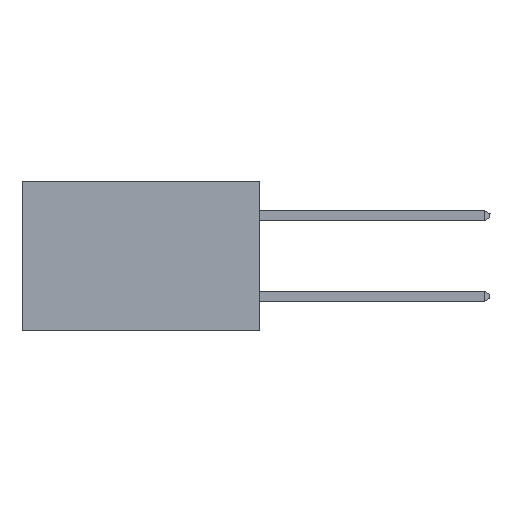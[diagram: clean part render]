
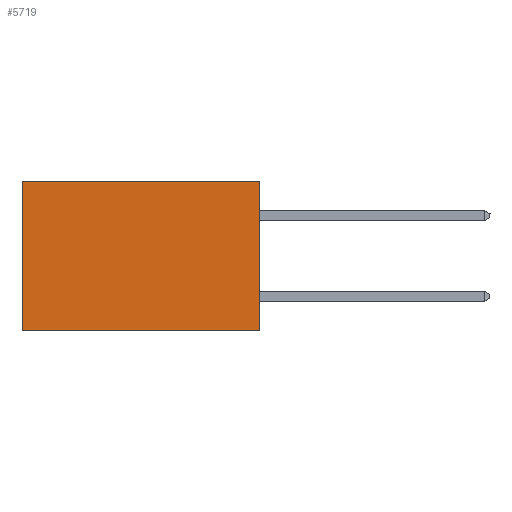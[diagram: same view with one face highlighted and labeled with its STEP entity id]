
A CAD part, left-side view. The second image highlights one B-rep face of the part: STEP entity #5719.
In plain terms, the highlighted planar face has unit normal (-1, 0, 0).
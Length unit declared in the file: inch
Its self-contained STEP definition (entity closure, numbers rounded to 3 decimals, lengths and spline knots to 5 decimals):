
#597 = CARTESIAN_POINT ( 'NONE',  ( 0.277, 0., -0.37 ) ) ;
#754 = LINE ( 'NONE', #7205, #15923 ) ;
#850 = CARTESIAN_POINT ( 'NONE',  ( 0.277, 0., -0.37 ) ) ;
#2019 = DIRECTION ( 'NONE',  ( 0., 1., 0. ) ) ;
#2414 = CARTESIAN_POINT ( 'NONE',  ( 0.277, 0.59, -0.37 ) ) ;
#2562 = EDGE_CURVE ( 'NONE', #7016, #13449, #12896, .T. ) ;
#3403 = VECTOR ( 'NONE', #2019, 39.37008 ) ;
#3607 = CARTESIAN_POINT ( 'NONE',  ( 0.277, 0.59, -0.37 ) ) ;
#5714 = VERTEX_POINT ( 'NONE', #13468 ) ;
#5719 = ADVANCED_FACE ( 'NONE', ( #14705 ), #13391, .F. ) ;
#5927 = VECTOR ( 'NONE', #16769, 39.37008 ) ;
#7016 = VERTEX_POINT ( 'NONE', #7951 ) ;
#7205 = CARTESIAN_POINT ( 'NONE',  ( 0.277, 0., 0. ) ) ;
#7951 = CARTESIAN_POINT ( 'NONE',  ( 0.277, 0.59, 0. ) ) ;
#8186 = VECTOR ( 'NONE', #18211, 39.37008 ) ;
#11055 = LINE ( 'NONE', #597, #3403 ) ;
#11628 = EDGE_CURVE ( 'NONE', #5714, #16786, #13521, .T. ) ;
#11738 = EDGE_CURVE ( 'NONE', #5714, #7016, #754, .T. ) ;
#11986 = ORIENTED_EDGE ( 'NONE', *, *, #12000, .F. ) ;
#12000 = EDGE_CURVE ( 'NONE', #16786, #13449, #11055, .T. ) ;
#12896 = LINE ( 'NONE', #3607, #8186 ) ;
#13329 = DIRECTION ( 'NONE',  ( 0., 0., -1. ) ) ;
#13344 = DIRECTION ( 'NONE',  ( 1., 0., 0. ) ) ;
#13391 = PLANE ( 'NONE',  #15771 ) ;
#13449 = VERTEX_POINT ( 'NONE', #2414 ) ;
#13468 = CARTESIAN_POINT ( 'NONE',  ( 0.277, 0., 0. ) ) ;
#13521 = LINE ( 'NONE', #13991, #5927 ) ;
#13599 = CARTESIAN_POINT ( 'NONE',  ( 0.277, 0., -0.37 ) ) ;
#13991 = CARTESIAN_POINT ( 'NONE',  ( 0.277, 0., -0.37 ) ) ;
#14416 = ORIENTED_EDGE ( 'NONE', *, *, #11738, .T. ) ;
#14562 = ORIENTED_EDGE ( 'NONE', *, *, #11628, .F. ) ;
#14705 = FACE_OUTER_BOUND ( 'NONE', #15480, .T. ) ;
#15480 = EDGE_LOOP ( 'NONE', ( #17974, #11986, #14562, #14416 ) ) ;
#15686 = DIRECTION ( 'NONE',  ( 0., 1., 0. ) ) ;
#15771 = AXIS2_PLACEMENT_3D ( 'NONE', #13599, #13344, #13329 ) ;
#15923 = VECTOR ( 'NONE', #15686, 39.37008 ) ;
#16769 = DIRECTION ( 'NONE',  ( 0., 0., -1. ) ) ;
#16786 = VERTEX_POINT ( 'NONE', #850 ) ;
#17974 = ORIENTED_EDGE ( 'NONE', *, *, #2562, .T. ) ;
#18211 = DIRECTION ( 'NONE',  ( 0., 0., -1. ) ) ;
